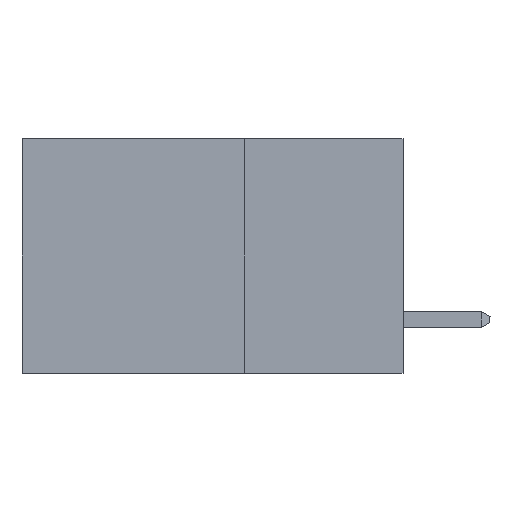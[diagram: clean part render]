
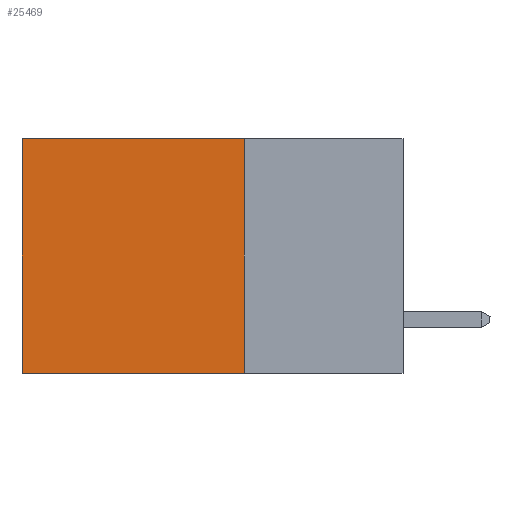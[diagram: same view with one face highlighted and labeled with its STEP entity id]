
A CAD part, left-side view. The second image highlights one B-rep face of the part: STEP entity #25469.
In plain terms, the highlighted planar face has unit normal (-1, 0, 0).
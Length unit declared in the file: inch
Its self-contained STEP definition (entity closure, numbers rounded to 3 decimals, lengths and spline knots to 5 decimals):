
#1398 = DIRECTION ( 'NONE',  ( 0., 0., -1. ) ) ;
#1640 = VERTEX_POINT ( 'NONE', #17546 ) ;
#4237 = DIRECTION ( 'NONE',  ( 0., 1., 0. ) ) ;
#6582 = LINE ( 'NONE', #9127, #25247 ) ;
#7549 = VECTOR ( 'NONE', #12355, 39.37008 ) ;
#7752 = DIRECTION ( 'NONE',  ( 0., 0., -1. ) ) ;
#8361 = LINE ( 'NONE', #9564, #11911 ) ;
#9127 = CARTESIAN_POINT ( 'NONE',  ( 0.2875, 0.25, 0. ) ) ;
#9152 = CARTESIAN_POINT ( 'NONE',  ( 0.2875, 0.25, 0. ) ) ;
#9564 = CARTESIAN_POINT ( 'NONE',  ( 0.2875, 0.25, -0.37 ) ) ;
#10431 = EDGE_CURVE ( 'NONE', #16822, #14921, #16428, .T. ) ;
#11897 = CARTESIAN_POINT ( 'NONE',  ( 0.2875, 0.6, 0. ) ) ;
#11911 = VECTOR ( 'NONE', #4237, 39.37008 ) ;
#12355 = DIRECTION ( 'NONE',  ( 0., 0., -1. ) ) ;
#12459 = CARTESIAN_POINT ( 'NONE',  ( 0.2875, 0.25, 0. ) ) ;
#14017 = DIRECTION ( 'NONE',  ( 1., 0., 0. ) ) ;
#14921 = VERTEX_POINT ( 'NONE', #21361 ) ;
#15654 = VECTOR ( 'NONE', #7752, 39.37008 ) ;
#16428 = LINE ( 'NONE', #18064, #15654 ) ;
#16822 = VERTEX_POINT ( 'NONE', #11897 ) ;
#16904 = EDGE_CURVE ( 'NONE', #21332, #14921, #8361, .T. ) ;
#17546 = CARTESIAN_POINT ( 'NONE',  ( 0.2875, 0.25, 0. ) ) ;
#18064 = CARTESIAN_POINT ( 'NONE',  ( 0.2875, 0.6, 0. ) ) ;
#18661 = LINE ( 'NONE', #12459, #7549 ) ;
#19350 = CARTESIAN_POINT ( 'NONE',  ( 0.2875, 0.25, -0.37 ) ) ;
#21332 = VERTEX_POINT ( 'NONE', #19350 ) ;
#21361 = CARTESIAN_POINT ( 'NONE',  ( 0.2875, 0.6, -0.37 ) ) ;
#21515 = EDGE_CURVE ( 'NONE', #1640, #21332, #18661, .T. ) ;
#21546 = DIRECTION ( 'NONE',  ( 0., 1., 0. ) ) ;
#22744 = ORIENTED_EDGE ( 'NONE', *, *, #26889, .T. ) ;
#23310 = EDGE_LOOP ( 'NONE', ( #27272, #30350, #27961, #22744 ) ) ;
#24472 = PLANE ( 'NONE',  #31311 ) ;
#25247 = VECTOR ( 'NONE', #21546, 39.37008 ) ;
#25469 = ADVANCED_FACE ( 'NONE', ( #27132 ), #24472, .F. ) ;
#26889 = EDGE_CURVE ( 'NONE', #1640, #16822, #6582, .T. ) ;
#27132 = FACE_OUTER_BOUND ( 'NONE', #23310, .T. ) ;
#27272 = ORIENTED_EDGE ( 'NONE', *, *, #10431, .T. ) ;
#27961 = ORIENTED_EDGE ( 'NONE', *, *, #21515, .F. ) ;
#30350 = ORIENTED_EDGE ( 'NONE', *, *, #16904, .F. ) ;
#31311 = AXIS2_PLACEMENT_3D ( 'NONE', #9152, #14017, #1398 ) ;
